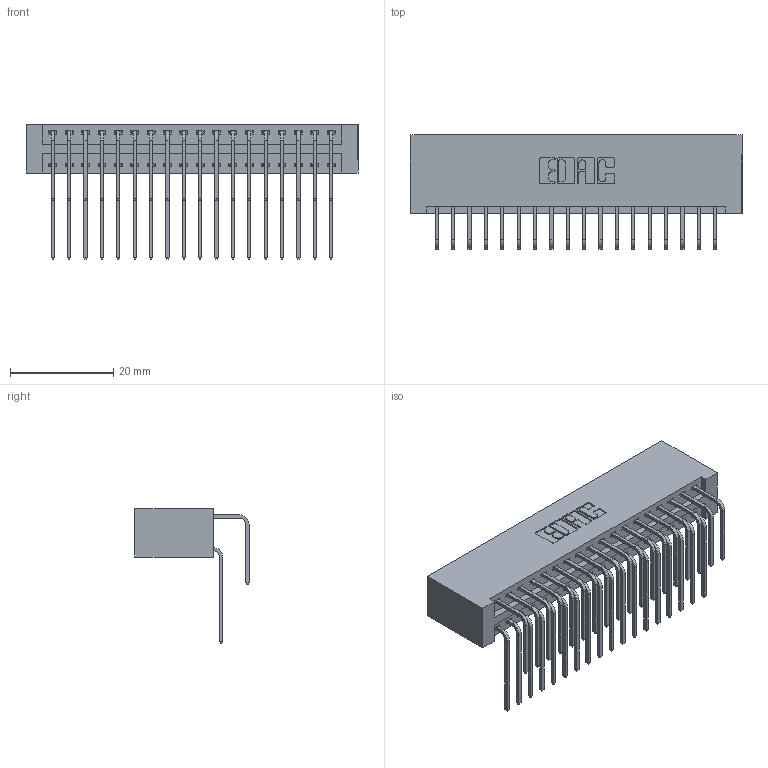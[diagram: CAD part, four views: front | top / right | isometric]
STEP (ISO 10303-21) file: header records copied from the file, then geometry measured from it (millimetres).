
FILE_DESCRIPTION (( 'STEP AP203' ), '1' );
FILE_NAME ('346-036-558-201.STEP', '2018-08-24T02:26:22', ( '' ), ( '' ), 'SwSTEP 2.0', 'SolidWorks 2016', '' );
FILE_SCHEMA (( 'CONFIG_CONTROL_DESIGN' ));
Length unit declared in the file: inch
Products named in the file (4): 345-292-001_558 Tail - 2; 346-036-558-201; 346 Part_No Mounting Lugs; 345-292-001_558 559 Tail - 1
Assembly tree (37 placements, depth 2):
  346-036-558-201
    346 Part_No Mounting Lugs
    345-292-001_558 559 Tail - 1  x18
    345-292-001_558 Tail - 2  x18
Bounding box: 64.39 x 22.16 x 26.16 mm (x, y, z)
Volume: 6873.3 mm3; surface area: 10230 mm2
Topology: 37 solids, 37 shells, 2058 faces, 6101 edges, 4018 vertices
Faces by surface type: plane 1404, cylinder 654
Entity records: 16485 total; most frequent: CARTESIAN_POINT 2799, ORIENTED_EDGE 2682, DIRECTION 2485, EDGE_CURVE 1341, LINE 1105, VECTOR 1105, VERTEX_POINT 890, AXIS2_PLACEMENT_3D 690
